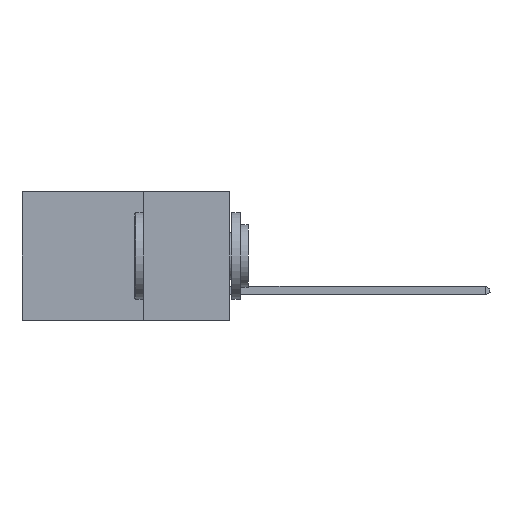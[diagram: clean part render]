
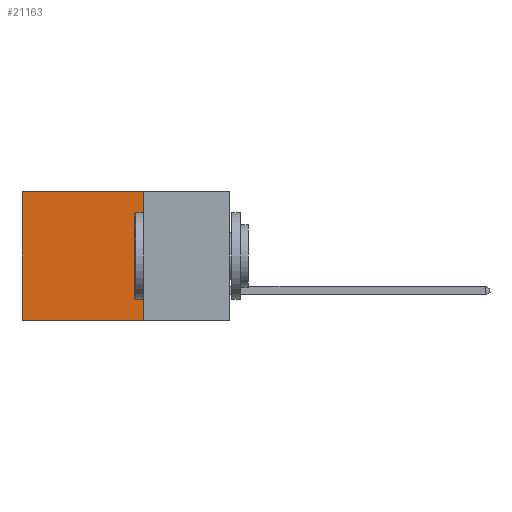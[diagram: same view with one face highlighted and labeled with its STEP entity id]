
A CAD part, left-side view. The second image highlights one B-rep face of the part: STEP entity #21163.
In plain terms, the highlighted planar face has unit normal (-1, 0, 0).
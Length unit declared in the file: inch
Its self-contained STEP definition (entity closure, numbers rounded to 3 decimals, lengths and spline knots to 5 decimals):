
#760 = ORIENTED_EDGE ( 'NONE', *, *, #7950, .T. ) ;
#2327 = CARTESIAN_POINT ( 'NONE',  ( 0.298, 0.25, 0. ) ) ;
#2738 = AXIS2_PLACEMENT_3D ( 'NONE', #25310, #15708, #10917 ) ;
#6806 = VECTOR ( 'NONE', #12158, 39.37008 ) ;
#6881 = ORIENTED_EDGE ( 'NONE', *, *, #22387, .T. ) ;
#7234 = EDGE_CURVE ( 'NONE', #30676, #13756, #18767, .T. ) ;
#7934 = VECTOR ( 'NONE', #21581, 39.37008 ) ;
#7950 = EDGE_CURVE ( 'NONE', #30676, #12819, #22220, .T. ) ;
#8229 = VERTEX_POINT ( 'NONE', #8770 ) ;
#8770 = CARTESIAN_POINT ( 'NONE',  ( 0.298, 0.6, -0.37 ) ) ;
#10917 = DIRECTION ( 'NONE',  ( 0., 0., -1. ) ) ;
#11577 = DIRECTION ( 'NONE',  ( 0., 0., -1. ) ) ;
#12158 = DIRECTION ( 'NONE',  ( 0., 1., 0. ) ) ;
#12819 = VERTEX_POINT ( 'NONE', #17425 ) ;
#13143 = PLANE ( 'NONE',  #2738 ) ;
#13756 = VERTEX_POINT ( 'NONE', #27463 ) ;
#14148 = EDGE_LOOP ( 'NONE', ( #6881, #29639, #19410, #760 ) ) ;
#15110 = LINE ( 'NONE', #19369, #7934 ) ;
#15708 = DIRECTION ( 'NONE',  ( 1., 0., 0. ) ) ;
#16267 = LINE ( 'NONE', #30766, #25622 ) ;
#17164 = VECTOR ( 'NONE', #26342, 39.37008 ) ;
#17425 = CARTESIAN_POINT ( 'NONE',  ( 0.298, 0.6, 0. ) ) ;
#18767 = LINE ( 'NONE', #21759, #17164 ) ;
#18943 = EDGE_CURVE ( 'NONE', #13756, #8229, #15110, .T. ) ;
#19369 = CARTESIAN_POINT ( 'NONE',  ( 0.298, 0.25, -0.37 ) ) ;
#19410 = ORIENTED_EDGE ( 'NONE', *, *, #7234, .F. ) ;
#21163 = ADVANCED_FACE ( 'NONE', ( #22385 ), #13143, .F. ) ;
#21581 = DIRECTION ( 'NONE',  ( 0., 1., 0. ) ) ;
#21759 = CARTESIAN_POINT ( 'NONE',  ( 0.298, 0.25, 0. ) ) ;
#22111 = CARTESIAN_POINT ( 'NONE',  ( 0.298, 0.25, 0. ) ) ;
#22220 = LINE ( 'NONE', #2327, #6806 ) ;
#22385 = FACE_OUTER_BOUND ( 'NONE', #14148, .T. ) ;
#22387 = EDGE_CURVE ( 'NONE', #12819, #8229, #16267, .T. ) ;
#25310 = CARTESIAN_POINT ( 'NONE',  ( 0.298, 0.25, 0. ) ) ;
#25622 = VECTOR ( 'NONE', #11577, 39.37008 ) ;
#26342 = DIRECTION ( 'NONE',  ( 0., 0., -1. ) ) ;
#27463 = CARTESIAN_POINT ( 'NONE',  ( 0.298, 0.25, -0.37 ) ) ;
#29639 = ORIENTED_EDGE ( 'NONE', *, *, #18943, .F. ) ;
#30676 = VERTEX_POINT ( 'NONE', #22111 ) ;
#30766 = CARTESIAN_POINT ( 'NONE',  ( 0.298, 0.6, 0. ) ) ;
